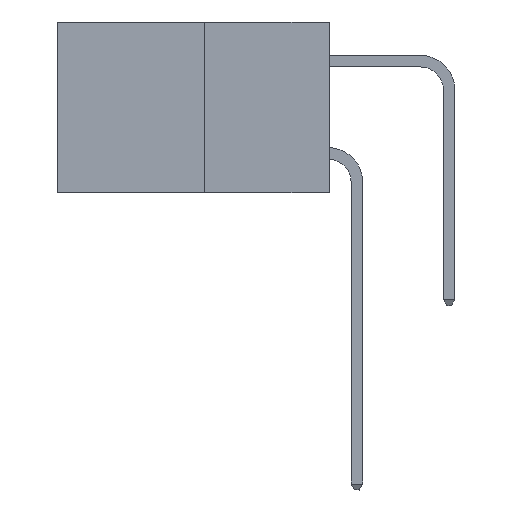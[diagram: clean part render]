
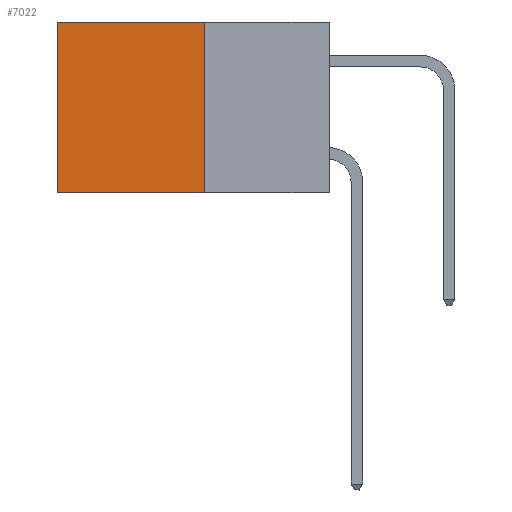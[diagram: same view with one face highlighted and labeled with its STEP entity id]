
A CAD part, left-side view. The second image highlights one B-rep face of the part: STEP entity #7022.
In plain terms, the highlighted planar face has unit normal (-1, 0, 0).
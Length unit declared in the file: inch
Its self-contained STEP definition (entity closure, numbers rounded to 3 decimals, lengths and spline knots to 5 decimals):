
#402 = EDGE_CURVE ( 'NONE', #3801, #18495, #15474, .T. ) ;
#2393 = DIRECTION ( 'NONE',  ( 0., 1., 0. ) ) ;
#2502 = VECTOR ( 'NONE', #16142, 39.37008 ) ;
#3548 = LINE ( 'NONE', #10424, #11607 ) ;
#3801 = VERTEX_POINT ( 'NONE', #8881 ) ;
#5214 = DIRECTION ( 'NONE',  ( 0., 0., -1. ) ) ;
#5218 = DIRECTION ( 'NONE',  ( 1., 0., 0. ) ) ;
#5308 = CARTESIAN_POINT ( 'NONE',  ( 0.277, 0.27, -0.37 ) ) ;
#5327 = PLANE ( 'NONE',  #11339 ) ;
#5918 = FACE_OUTER_BOUND ( 'NONE', #20828, .T. ) ;
#6165 = ORIENTED_EDGE ( 'NONE', *, *, #402, .T. ) ;
#7022 = ADVANCED_FACE ( 'NONE', ( #5918 ), #5327, .F. ) ;
#7630 = DIRECTION ( 'NONE',  ( 0., 0., -1. ) ) ;
#7758 = CARTESIAN_POINT ( 'NONE',  ( 0.277, 0.59, -0.37 ) ) ;
#8695 = EDGE_CURVE ( 'NONE', #18495, #12769, #12606, .T. ) ;
#8707 = ORIENTED_EDGE ( 'NONE', *, *, #11088, .F. ) ;
#8881 = CARTESIAN_POINT ( 'NONE',  ( 0.277, 0.27, 0. ) ) ;
#9521 = CARTESIAN_POINT ( 'NONE',  ( 0.277, 0.59, -0.37 ) ) ;
#10218 = EDGE_CURVE ( 'NONE', #3801, #13427, #16065, .T. ) ;
#10424 = CARTESIAN_POINT ( 'NONE',  ( 0.277, 0.27, -0.37 ) ) ;
#11088 = EDGE_CURVE ( 'NONE', #13427, #12769, #3548, .T. ) ;
#11136 = VECTOR ( 'NONE', #13094, 39.37008 ) ;
#11339 = AXIS2_PLACEMENT_3D ( 'NONE', #5308, #5218, #5214 ) ;
#11607 = VECTOR ( 'NONE', #2393, 39.37008 ) ;
#12606 = LINE ( 'NONE', #7758, #16994 ) ;
#12769 = VERTEX_POINT ( 'NONE', #9521 ) ;
#13094 = DIRECTION ( 'NONE',  ( 0., 0., -1. ) ) ;
#13427 = VERTEX_POINT ( 'NONE', #17643 ) ;
#14286 = ORIENTED_EDGE ( 'NONE', *, *, #10218, .F. ) ;
#15474 = LINE ( 'NONE', #19790, #2502 ) ;
#16065 = LINE ( 'NONE', #17966, #11136 ) ;
#16142 = DIRECTION ( 'NONE',  ( 0., 1., 0. ) ) ;
#16994 = VECTOR ( 'NONE', #7630, 39.37008 ) ;
#17022 = ORIENTED_EDGE ( 'NONE', *, *, #8695, .T. ) ;
#17643 = CARTESIAN_POINT ( 'NONE',  ( 0.277, 0.27, -0.37 ) ) ;
#17966 = CARTESIAN_POINT ( 'NONE',  ( 0.277, 0.27, -0.37 ) ) ;
#18495 = VERTEX_POINT ( 'NONE', #18546 ) ;
#18546 = CARTESIAN_POINT ( 'NONE',  ( 0.277, 0.59, 0. ) ) ;
#19790 = CARTESIAN_POINT ( 'NONE',  ( 0.277, 0.27, 0. ) ) ;
#20828 = EDGE_LOOP ( 'NONE', ( #17022, #8707, #14286, #6165 ) ) ;
